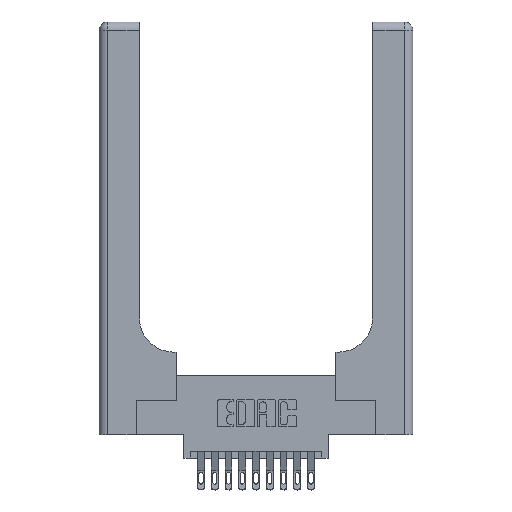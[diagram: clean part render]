
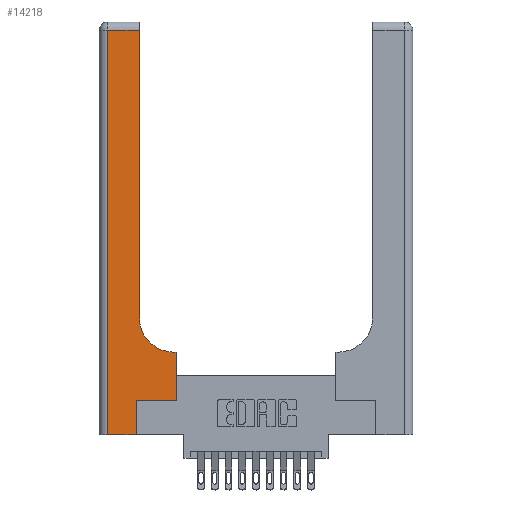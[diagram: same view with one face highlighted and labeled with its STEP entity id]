
A CAD part, top view. The second image highlights one B-rep face of the part: STEP entity #14218.
In plain terms, the highlighted planar face has unit normal (0, 0, 1).
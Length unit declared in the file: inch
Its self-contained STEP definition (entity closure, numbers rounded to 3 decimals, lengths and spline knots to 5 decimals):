
#300 = DIRECTION ( 'NONE',  ( -1., 0., 0. ) ) ;
#540 = VECTOR ( 'NONE', #5903, 39.37008 ) ;
#959 = CARTESIAN_POINT ( 'NONE',  ( 0.269, 0.25, 0.37 ) ) ;
#1278 = AXIS2_PLACEMENT_3D ( 'NONE', #2080, #16796, #16680 ) ;
#1388 = VECTOR ( 'NONE', #6074, 39.37008 ) ;
#1870 = CARTESIAN_POINT ( 'NONE',  ( 0.5585, 0.25, 0.37 ) ) ;
#1978 = VECTOR ( 'NONE', #11791, 39.37008 ) ;
#2080 = CARTESIAN_POINT ( 'NONE',  ( 0., 3., 0.37 ) ) ;
#2092 = CARTESIAN_POINT ( 'NONE',  ( 0.06, 2.94, 0.37 ) ) ;
#2227 = DIRECTION ( 'NONE',  ( 1., 0., 0. ) ) ;
#2633 = ORIENTED_EDGE ( 'NONE', *, *, #14154, .T. ) ;
#3242 = LINE ( 'NONE', #4083, #1978 ) ;
#3917 = ORIENTED_EDGE ( 'NONE', *, *, #6453, .T. ) ;
#4024 = ORIENTED_EDGE ( 'NONE', *, *, #8848, .T. ) ;
#4083 = CARTESIAN_POINT ( 'NONE',  ( 0., 0., 0.37 ) ) ;
#4561 = CARTESIAN_POINT ( 'NONE',  ( 0.5585, 0.6, 0.37 ) ) ;
#4873 = EDGE_CURVE ( 'NONE', #6667, #6101, #16386, .T. ) ;
#4892 = FACE_OUTER_BOUND ( 'NONE', #10155, .T. ) ;
#4942 = LINE ( 'NONE', #6366, #9289 ) ;
#5012 = VERTEX_POINT ( 'NONE', #16814 ) ;
#5017 = CARTESIAN_POINT ( 'NONE',  ( 0.06, 3., 0.37 ) ) ;
#5038 = ORIENTED_EDGE ( 'NONE', *, *, #13915, .T. ) ;
#5312 = CARTESIAN_POINT ( 'NONE',  ( 0.2915, 2.94, 0.37 ) ) ;
#5846 = CARTESIAN_POINT ( 'NONE',  ( 0., 2.94, 0.37 ) ) ;
#5854 = CARTESIAN_POINT ( 'NONE',  ( 0.5585, 0.25, 0.37 ) ) ;
#5903 = DIRECTION ( 'NONE',  ( -1., 0., 0. ) ) ;
#6074 = DIRECTION ( 'NONE',  ( 0., 1., 0. ) ) ;
#6101 = VERTEX_POINT ( 'NONE', #1870 ) ;
#6220 = VERTEX_POINT ( 'NONE', #2092 ) ;
#6339 = EDGE_CURVE ( 'NONE', #7033, #7229, #8473, .T. ) ;
#6356 = DIRECTION ( 'NONE',  ( 0., -1., 0. ) ) ;
#6366 = CARTESIAN_POINT ( 'NONE',  ( 0.269, 0., 0.37 ) ) ;
#6453 = EDGE_CURVE ( 'NONE', #5012, #6667, #4942, .T. ) ;
#6667 = VERTEX_POINT ( 'NONE', #12520 ) ;
#6781 = LINE ( 'NONE', #5846, #540 ) ;
#6845 = CARTESIAN_POINT ( 'NONE',  ( 0.2915, 0.85, 0.37 ) ) ;
#7033 = VERTEX_POINT ( 'NONE', #6845 ) ;
#7048 = CARTESIAN_POINT ( 'NONE',  ( 0.5415, 0.85, 0.37 ) ) ;
#7080 = ORIENTED_EDGE ( 'NONE', *, *, #9589, .T. ) ;
#7211 = LINE ( 'NONE', #5017, #13163 ) ;
#7212 = VERTEX_POINT ( 'NONE', #4561 ) ;
#7229 = VERTEX_POINT ( 'NONE', #5312 ) ;
#8473 = LINE ( 'NONE', #16585, #1388 ) ;
#8495 = CARTESIAN_POINT ( 'NONE',  ( 0.06, 0., 0.37 ) ) ;
#8848 = EDGE_CURVE ( 'NONE', #9388, #7033, #15208, .T. ) ;
#9148 = ORIENTED_EDGE ( 'NONE', *, *, #6339, .T. ) ;
#9171 = ORIENTED_EDGE ( 'NONE', *, *, #10757, .T. ) ;
#9289 = VECTOR ( 'NONE', #15602, 39.37008 ) ;
#9388 = VERTEX_POINT ( 'NONE', #9476 ) ;
#9476 = CARTESIAN_POINT ( 'NONE',  ( 0.5415, 0.6, 0.37 ) ) ;
#9588 = LINE ( 'NONE', #5854, #13925 ) ;
#9589 = EDGE_CURVE ( 'NONE', #6101, #7212, #9588, .T. ) ;
#10155 = EDGE_LOOP ( 'NONE', ( #9148, #2633, #15177, #5038, #3917, #11777, #7080, #9171, #4024 ) ) ;
#10384 = LINE ( 'NONE', #15997, #11430 ) ;
#10550 = AXIS2_PLACEMENT_3D ( 'NONE', #7048, #11020, #2227 ) ;
#10757 = EDGE_CURVE ( 'NONE', #7212, #9388, #10384, .T. ) ;
#11020 = DIRECTION ( 'NONE',  ( 0., 0., -1. ) ) ;
#11430 = VECTOR ( 'NONE', #300, 39.37008 ) ;
#11777 = ORIENTED_EDGE ( 'NONE', *, *, #4873, .T. ) ;
#11791 = DIRECTION ( 'NONE',  ( 1., 0., 0. ) ) ;
#12520 = CARTESIAN_POINT ( 'NONE',  ( 0.269, 0.25, 0.37 ) ) ;
#12592 = VERTEX_POINT ( 'NONE', #8495 ) ;
#12872 = DIRECTION ( 'NONE',  ( 1., 0., 0. ) ) ;
#13163 = VECTOR ( 'NONE', #6356, 39.37008 ) ;
#13747 = PLANE ( 'NONE',  #1278 ) ;
#13915 = EDGE_CURVE ( 'NONE', #12592, #5012, #3242, .T. ) ;
#13925 = VECTOR ( 'NONE', #16426, 39.37008 ) ;
#14154 = EDGE_CURVE ( 'NONE', #7229, #6220, #6781, .T. ) ;
#14218 = ADVANCED_FACE ( 'NONE', ( #4892 ), #13747, .F. ) ;
#14365 = EDGE_CURVE ( 'NONE', #6220, #12592, #7211, .T. ) ;
#15177 = ORIENTED_EDGE ( 'NONE', *, *, #14365, .T. ) ;
#15208 = CIRCLE ( 'NONE', #10550, 0.25 ) ;
#15602 = DIRECTION ( 'NONE',  ( 0., 1., 0. ) ) ;
#15997 = CARTESIAN_POINT ( 'NONE',  ( 0.2915, 0.6, 0.37 ) ) ;
#16386 = LINE ( 'NONE', #959, #16574 ) ;
#16426 = DIRECTION ( 'NONE',  ( 0., 1., 0. ) ) ;
#16574 = VECTOR ( 'NONE', #12872, 39.37008 ) ;
#16585 = CARTESIAN_POINT ( 'NONE',  ( 0.2915, 3., 0.37 ) ) ;
#16680 = DIRECTION ( 'NONE',  ( -1., 0., 0. ) ) ;
#16796 = DIRECTION ( 'NONE',  ( 0., 0., -1. ) ) ;
#16814 = CARTESIAN_POINT ( 'NONE',  ( 0.269, 0., 0.37 ) ) ;
